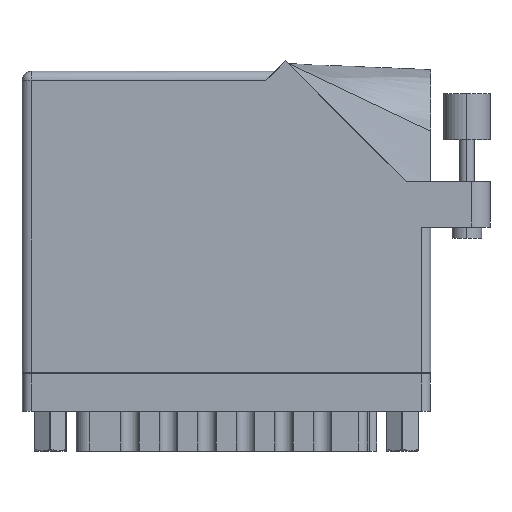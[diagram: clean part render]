
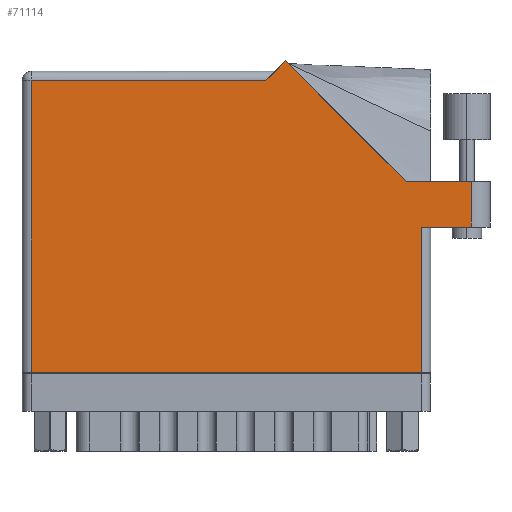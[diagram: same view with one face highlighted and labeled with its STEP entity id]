
A CAD part, front view. The second image highlights one B-rep face of the part: STEP entity #71114.
In plain terms, the highlighted face is planar.
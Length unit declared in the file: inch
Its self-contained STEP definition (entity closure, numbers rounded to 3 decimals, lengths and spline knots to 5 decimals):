
#3528 = CARTESIAN_POINT ( 'NONE',  ( 1.705, 2.03, 0. ) ) ;
#3570 = VERTEX_POINT ( 'NONE', #52192 ) ;
#5272 = DIRECTION ( 'NONE',  ( -1., 0., 0. ) ) ;
#7096 = VERTEX_POINT ( 'NONE', #87056 ) ;
#8086 = PLANE ( 'NONE',  #69795 ) ;
#10671 = CARTESIAN_POINT ( 'NONE',  ( 3.03, 1.287, 0. ) ) ;
#11583 = VECTOR ( 'NONE', #76080, 39.37008 ) ;
#12087 = EDGE_LOOP ( 'NONE', ( #19856, #45822, #41842, #52104, #83285, #69453, #67235, #91534, #60464 ) ) ;
#13273 = CARTESIAN_POINT ( 'NONE',  ( 2.693, 0., 0. ) ) ;
#14243 = VECTOR ( 'NONE', #25681, 39.37008 ) ;
#15116 = CARTESIAN_POINT ( 'NONE',  ( 2.58942, 1.287, 0. ) ) ;
#16468 = DIRECTION ( 'NONE',  ( -1., 0., 0. ) ) ;
#17286 = DIRECTION ( 'NONE',  ( 0., 1., 0. ) ) ;
#18100 = VECTOR ( 'NONE', #99585, 39.37008 ) ;
#19856 = ORIENTED_EDGE ( 'NONE', *, *, #50482, .T. ) ;
#20234 = VECTOR ( 'NONE', #25260, 39.37008 ) ;
#20266 = LINE ( 'NONE', #63944, #99618 ) ;
#20479 = DIRECTION ( 'NONE',  ( 1., 0., 0. ) ) ;
#25260 = DIRECTION ( 'NONE',  ( -0.707, 0.707, 0. ) ) ;
#25389 = EDGE_CURVE ( 'NONE', #56528, #3570, #75564, .T. ) ;
#25681 = DIRECTION ( 'NONE',  ( -0.707, -0.707, 0. ) ) ;
#26340 = VECTOR ( 'NONE', #85614, 39.37008 ) ;
#26393 = VECTOR ( 'NONE', #80080, 39.37008 ) ;
#28790 = LINE ( 'NONE', #36771, #26393 ) ;
#30142 = VERTEX_POINT ( 'NONE', #13273 ) ;
#30204 = LINE ( 'NONE', #98088, #91512 ) ;
#33762 = LINE ( 'NONE', #53865, #18100 ) ;
#34922 = EDGE_CURVE ( 'NONE', #48489, #30142, #38006, .T. ) ;
#36524 = EDGE_CURVE ( 'NONE', #92267, #91178, #28790, .T. ) ;
#36771 = CARTESIAN_POINT ( 'NONE',  ( 3.155, 1.287, 0. ) ) ;
#38006 = LINE ( 'NONE', #67370, #11583 ) ;
#39418 = CARTESIAN_POINT ( 'NONE',  ( 3.03, 0.98, 0. ) ) ;
#40100 = CARTESIAN_POINT ( 'NONE',  ( 1.77571, 2.10071, 0. ) ) ;
#40226 = CARTESIAN_POINT ( 'NONE',  ( 1.643, 1.968, 0. ) ) ;
#41842 = ORIENTED_EDGE ( 'NONE', *, *, #36524, .T. ) ;
#45394 = VERTEX_POINT ( 'NONE', #40100 ) ;
#45585 = EDGE_CURVE ( 'NONE', #45394, #56528, #74286, .T. ) ;
#45822 = ORIENTED_EDGE ( 'NONE', *, *, #71818, .T. ) ;
#48489 = VERTEX_POINT ( 'NONE', #68565 ) ;
#50482 = EDGE_CURVE ( 'NONE', #7096, #79215, #30204, .T. ) ;
#52104 = ORIENTED_EDGE ( 'NONE', *, *, #67995, .T. ) ;
#52192 = CARTESIAN_POINT ( 'NONE',  ( 0.062, 1.968, 0. ) ) ;
#53865 = CARTESIAN_POINT ( 'NONE',  ( 3.03, 1.287, 0. ) ) ;
#56528 = VERTEX_POINT ( 'NONE', #40226 ) ;
#59972 = CARTESIAN_POINT ( 'NONE',  ( 0., 1.968, 0. ) ) ;
#60464 = ORIENTED_EDGE ( 'NONE', *, *, #92722, .T. ) ;
#61795 = CARTESIAN_POINT ( 'NONE',  ( 0., 2.03, 0. ) ) ;
#62474 = DIRECTION ( 'NONE',  ( 0., 0., -1. ) ) ;
#63944 = CARTESIAN_POINT ( 'NONE',  ( 2.693, 0.98, 0. ) ) ;
#65940 = LINE ( 'NONE', #70300, #20234 ) ;
#66973 = EDGE_CURVE ( 'NONE', #3570, #48489, #92443, .T. ) ;
#67235 = ORIENTED_EDGE ( 'NONE', *, *, #66973, .T. ) ;
#67370 = CARTESIAN_POINT ( 'NONE',  ( 0., 0., 0. ) ) ;
#67995 = EDGE_CURVE ( 'NONE', #91178, #45394, #65940, .T. ) ;
#68368 = VECTOR ( 'NONE', #5272, 39.37008 ) ;
#68565 = CARTESIAN_POINT ( 'NONE',  ( 0.062, 0., 0. ) ) ;
#69453 = ORIENTED_EDGE ( 'NONE', *, *, #25389, .T. ) ;
#69795 = AXIS2_PLACEMENT_3D ( 'NONE', #61795, #62474, #16468 ) ;
#69849 = CARTESIAN_POINT ( 'NONE',  ( 0.062, 0., 0. ) ) ;
#70300 = CARTESIAN_POINT ( 'NONE',  ( 2.58942, 1.287, 0. ) ) ;
#71114 = ADVANCED_FACE ( 'NONE', ( #76021 ), #8086, .F. ) ;
#71818 = EDGE_CURVE ( 'NONE', #79215, #92267, #33762, .T. ) ;
#74286 = LINE ( 'NONE', #3528, #14243 ) ;
#75564 = LINE ( 'NONE', #59972, #68368 ) ;
#76021 = FACE_OUTER_BOUND ( 'NONE', #12087, .T. ) ;
#76080 = DIRECTION ( 'NONE',  ( 1., 0., 0. ) ) ;
#79215 = VERTEX_POINT ( 'NONE', #39418 ) ;
#80080 = DIRECTION ( 'NONE',  ( -1., 0., 0. ) ) ;
#83285 = ORIENTED_EDGE ( 'NONE', *, *, #45585, .T. ) ;
#85614 = DIRECTION ( 'NONE',  ( 0., -1., 0. ) ) ;
#87056 = CARTESIAN_POINT ( 'NONE',  ( 2.693, 0.98, 0. ) ) ;
#91178 = VERTEX_POINT ( 'NONE', #15116 ) ;
#91512 = VECTOR ( 'NONE', #20479, 39.37008 ) ;
#91534 = ORIENTED_EDGE ( 'NONE', *, *, #34922, .T. ) ;
#92267 = VERTEX_POINT ( 'NONE', #10671 ) ;
#92443 = LINE ( 'NONE', #69849, #26340 ) ;
#92722 = EDGE_CURVE ( 'NONE', #30142, #7096, #20266, .T. ) ;
#98088 = CARTESIAN_POINT ( 'NONE',  ( 2.755, 0.98, 0. ) ) ;
#99585 = DIRECTION ( 'NONE',  ( 0., 1., 0. ) ) ;
#99618 = VECTOR ( 'NONE', #17286, 39.37008 ) ;
